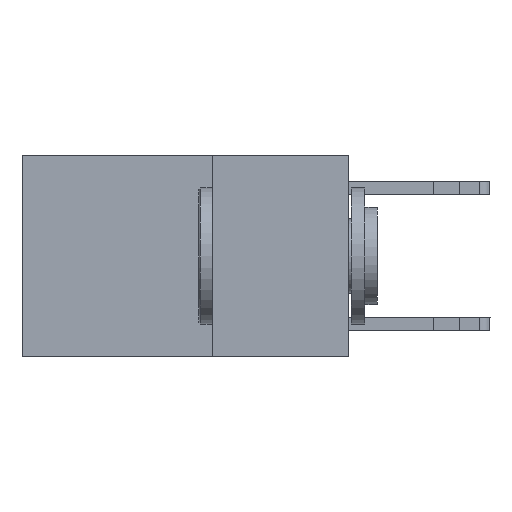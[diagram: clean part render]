
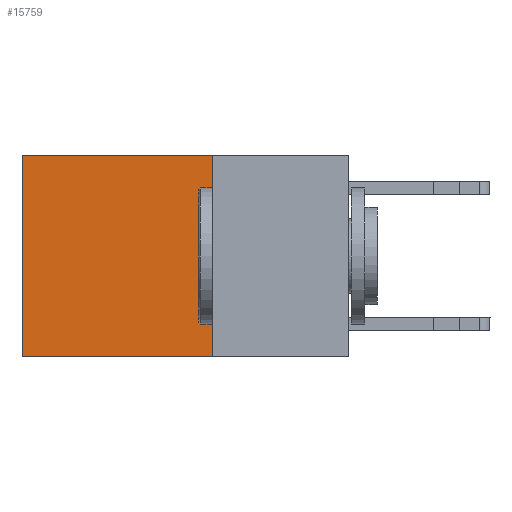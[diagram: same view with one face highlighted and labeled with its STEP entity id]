
A CAD part, left-side view. The second image highlights one B-rep face of the part: STEP entity #15759.
In plain terms, the highlighted planar face has unit normal (-1, 0, 0).
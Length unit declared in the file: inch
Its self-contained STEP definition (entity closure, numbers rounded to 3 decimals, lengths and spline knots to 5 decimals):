
#640 = VERTEX_POINT ( 'NONE', #15682 ) ;
#1090 = DIRECTION ( 'NONE',  ( 0., 0., -1. ) ) ;
#1222 = VECTOR ( 'NONE', #5143, 39.37008 ) ;
#1340 = CARTESIAN_POINT ( 'NONE',  ( 0.2625, 0.6, -0.37 ) ) ;
#1416 = AXIS2_PLACEMENT_3D ( 'NONE', #6183, #8516, #1090 ) ;
#1913 = EDGE_CURVE ( 'NONE', #5595, #14020, #13993, .T. ) ;
#2404 = DIRECTION ( 'NONE',  ( 0., 1., 0. ) ) ;
#2427 = ORIENTED_EDGE ( 'NONE', *, *, #1913, .F. ) ;
#2437 = FACE_OUTER_BOUND ( 'NONE', #7312, .T. ) ;
#3893 = CARTESIAN_POINT ( 'NONE',  ( 0.2625, 0.25, 0. ) ) ;
#3990 = ORIENTED_EDGE ( 'NONE', *, *, #8530, .T. ) ;
#5048 = DIRECTION ( 'NONE',  ( 0., 0., -1. ) ) ;
#5143 = DIRECTION ( 'NONE',  ( 0., 1., 0. ) ) ;
#5305 = LINE ( 'NONE', #3893, #7412 ) ;
#5595 = VERTEX_POINT ( 'NONE', #8714 ) ;
#6183 = CARTESIAN_POINT ( 'NONE',  ( 0.2625, 0.25, 0. ) ) ;
#7312 = EDGE_LOOP ( 'NONE', ( #3990, #2427, #10599, #8649 ) ) ;
#7412 = VECTOR ( 'NONE', #5048, 39.37008 ) ;
#7987 = LINE ( 'NONE', #11159, #13340 ) ;
#8516 = DIRECTION ( 'NONE',  ( 1., 0., 0. ) ) ;
#8530 = EDGE_CURVE ( 'NONE', #640, #14020, #12074, .T. ) ;
#8649 = ORIENTED_EDGE ( 'NONE', *, *, #11190, .T. ) ;
#8714 = CARTESIAN_POINT ( 'NONE',  ( 0.2625, 0.25, -0.37 ) ) ;
#8790 = VECTOR ( 'NONE', #14575, 39.37008 ) ;
#9391 = VERTEX_POINT ( 'NONE', #11518 ) ;
#9560 = CARTESIAN_POINT ( 'NONE',  ( 0.2625, 0.6, 0. ) ) ;
#10599 = ORIENTED_EDGE ( 'NONE', *, *, #11280, .F. ) ;
#11159 = CARTESIAN_POINT ( 'NONE',  ( 0.2625, 0.25, 0. ) ) ;
#11190 = EDGE_CURVE ( 'NONE', #9391, #640, #7987, .T. ) ;
#11280 = EDGE_CURVE ( 'NONE', #9391, #5595, #5305, .T. ) ;
#11518 = CARTESIAN_POINT ( 'NONE',  ( 0.2625, 0.25, 0. ) ) ;
#12074 = LINE ( 'NONE', #9560, #8790 ) ;
#12729 = PLANE ( 'NONE',  #1416 ) ;
#13340 = VECTOR ( 'NONE', #2404, 39.37008 ) ;
#13993 = LINE ( 'NONE', #14078, #1222 ) ;
#14020 = VERTEX_POINT ( 'NONE', #1340 ) ;
#14078 = CARTESIAN_POINT ( 'NONE',  ( 0.2625, 0.25, -0.37 ) ) ;
#14575 = DIRECTION ( 'NONE',  ( 0., 0., -1. ) ) ;
#15682 = CARTESIAN_POINT ( 'NONE',  ( 0.2625, 0.6, 0. ) ) ;
#15759 = ADVANCED_FACE ( 'NONE', ( #2437 ), #12729, .F. ) ;
